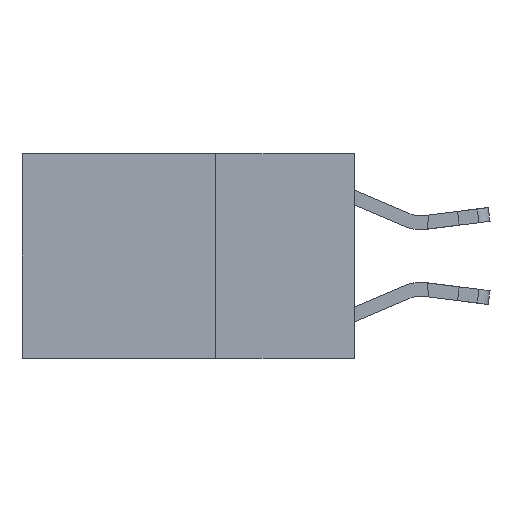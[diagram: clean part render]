
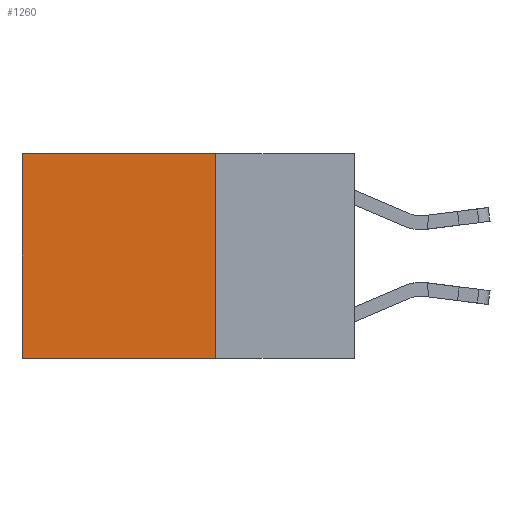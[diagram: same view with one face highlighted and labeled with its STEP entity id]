
A CAD part, left-side view. The second image highlights one B-rep face of the part: STEP entity #1260.
In plain terms, the highlighted planar face has unit normal (-1, 0, 0).
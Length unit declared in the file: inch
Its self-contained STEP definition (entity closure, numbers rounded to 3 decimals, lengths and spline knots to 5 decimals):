
#345 = DIRECTION ( 'NONE',  ( 1., 0., 0. ) ) ;
#791 = VERTEX_POINT ( 'NONE', #1719 ) ;
#796 = DIRECTION ( 'NONE',  ( 0., 0., -1. ) ) ;
#1260 = ADVANCED_FACE ( 'NONE', ( #14220 ), #2421, .F. ) ;
#1719 = CARTESIAN_POINT ( 'NONE',  ( 0.2625, 0.25, 0. ) ) ;
#2421 = PLANE ( 'NONE',  #10178 ) ;
#2634 = CARTESIAN_POINT ( 'NONE',  ( 0.2625, 0.6, 0. ) ) ;
#3596 = DIRECTION ( 'NONE',  ( 0., 0., -1. ) ) ;
#3660 = VECTOR ( 'NONE', #9592, 39.37008 ) ;
#4032 = CARTESIAN_POINT ( 'NONE',  ( 0.2625, 0.25, -0.37 ) ) ;
#4828 = CARTESIAN_POINT ( 'NONE',  ( 0.2625, 0.25, 0. ) ) ;
#5392 = VERTEX_POINT ( 'NONE', #14475 ) ;
#6346 = VECTOR ( 'NONE', #13228, 39.37008 ) ;
#6523 = VERTEX_POINT ( 'NONE', #14028 ) ;
#7206 = DIRECTION ( 'NONE',  ( 0., 0., -1. ) ) ;
#7217 = EDGE_LOOP ( 'NONE', ( #9003, #11268, #15162, #10125 ) ) ;
#7349 = LINE ( 'NONE', #2634, #8557 ) ;
#7612 = VERTEX_POINT ( 'NONE', #4032 ) ;
#8557 = VECTOR ( 'NONE', #7206, 39.37008 ) ;
#8839 = VECTOR ( 'NONE', #796, 39.37008 ) ;
#9003 = ORIENTED_EDGE ( 'NONE', *, *, #10674, .T. ) ;
#9282 = EDGE_CURVE ( 'NONE', #791, #5392, #12867, .T. ) ;
#9283 = CARTESIAN_POINT ( 'NONE',  ( 0.2625, 0.25, 0. ) ) ;
#9516 = CARTESIAN_POINT ( 'NONE',  ( 0.2625, 0.25, 0. ) ) ;
#9592 = DIRECTION ( 'NONE',  ( 0., 1., 0. ) ) ;
#9830 = EDGE_CURVE ( 'NONE', #7612, #6523, #13147, .T. ) ;
#10125 = ORIENTED_EDGE ( 'NONE', *, *, #9282, .T. ) ;
#10178 = AXIS2_PLACEMENT_3D ( 'NONE', #4828, #345, #3596 ) ;
#10674 = EDGE_CURVE ( 'NONE', #5392, #6523, #7349, .T. ) ;
#11268 = ORIENTED_EDGE ( 'NONE', *, *, #9830, .F. ) ;
#11476 = LINE ( 'NONE', #9283, #8839 ) ;
#11992 = CARTESIAN_POINT ( 'NONE',  ( 0.2625, 0.25, -0.37 ) ) ;
#12867 = LINE ( 'NONE', #9516, #3660 ) ;
#13147 = LINE ( 'NONE', #11992, #6346 ) ;
#13228 = DIRECTION ( 'NONE',  ( 0., 1., 0. ) ) ;
#14028 = CARTESIAN_POINT ( 'NONE',  ( 0.2625, 0.6, -0.37 ) ) ;
#14193 = EDGE_CURVE ( 'NONE', #791, #7612, #11476, .T. ) ;
#14220 = FACE_OUTER_BOUND ( 'NONE', #7217, .T. ) ;
#14475 = CARTESIAN_POINT ( 'NONE',  ( 0.2625, 0.6, 0. ) ) ;
#15162 = ORIENTED_EDGE ( 'NONE', *, *, #14193, .F. ) ;
